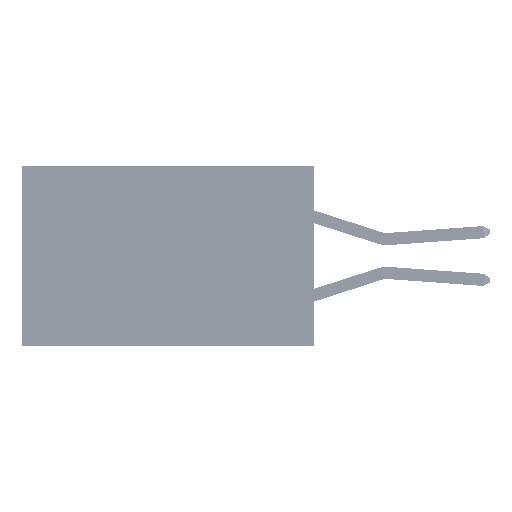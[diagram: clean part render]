
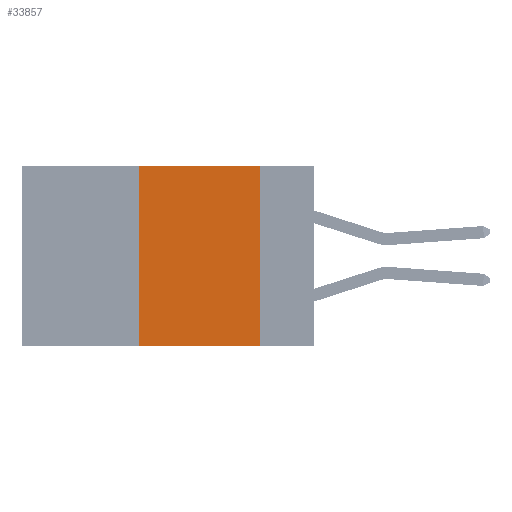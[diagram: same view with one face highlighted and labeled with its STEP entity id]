
A CAD part, left-side view. The second image highlights one B-rep face of the part: STEP entity #33857.
In plain terms, the highlighted planar face has unit normal (-1, 0, 0).
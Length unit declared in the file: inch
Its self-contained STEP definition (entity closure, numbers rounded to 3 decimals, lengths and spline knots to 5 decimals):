
#4185 = LINE ( 'NONE', #24525, #13109 ) ;
#5312 = VECTOR ( 'NONE', #49430, 39.37008 ) ;
#6240 = CARTESIAN_POINT ( 'NONE',  ( 0., 0.11, 0. ) ) ;
#9006 = ORIENTED_EDGE ( 'NONE', *, *, #12312, .T. ) ;
#10486 = EDGE_CURVE ( 'NONE', #29280, #26717, #4185, .T. ) ;
#10810 = EDGE_CURVE ( 'NONE', #26717, #48323, #37036, .T. ) ;
#11540 = DIRECTION ( 'NONE',  ( 1., 0., 0. ) ) ;
#12204 = VECTOR ( 'NONE', #24354, 39.37008 ) ;
#12312 = EDGE_CURVE ( 'NONE', #29280, #48264, #26581, .T. ) ;
#13109 = VECTOR ( 'NONE', #35706, 39.37008 ) ;
#14360 = CARTESIAN_POINT ( 'NONE',  ( 0., 0.11, 0. ) ) ;
#15136 = FACE_OUTER_BOUND ( 'NONE', #15821, .T. ) ;
#15810 = EDGE_CURVE ( 'NONE', #48323, #48264, #21415, .T. ) ;
#15821 = EDGE_LOOP ( 'NONE', ( #18045, #40813, #42378, #9006 ) ) ;
#18045 = ORIENTED_EDGE ( 'NONE', *, *, #15810, .F. ) ;
#20361 = CARTESIAN_POINT ( 'NONE',  ( 0., 0.36, 0. ) ) ;
#21415 = LINE ( 'NONE', #6240, #42325 ) ;
#23355 = CARTESIAN_POINT ( 'NONE',  ( 0., 0.6, -0.37 ) ) ;
#24354 = DIRECTION ( 'NONE',  ( 0., -1., 0. ) ) ;
#24525 = CARTESIAN_POINT ( 'NONE',  ( 0., 0.36, 0. ) ) ;
#24885 = CARTESIAN_POINT ( 'NONE',  ( 0., 0.11, -0.37 ) ) ;
#26581 = LINE ( 'NONE', #23355, #12204 ) ;
#26717 = VERTEX_POINT ( 'NONE', #20361 ) ;
#29280 = VERTEX_POINT ( 'NONE', #29823 ) ;
#29823 = CARTESIAN_POINT ( 'NONE',  ( 0., 0.36, -0.37 ) ) ;
#30083 = AXIS2_PLACEMENT_3D ( 'NONE', #37840, #11540, #30618 ) ;
#30618 = DIRECTION ( 'NONE',  ( 0., 0., -1. ) ) ;
#32639 = DIRECTION ( 'NONE',  ( 0., 0., -1. ) ) ;
#33857 = ADVANCED_FACE ( 'NONE', ( #15136 ), #40845, .F. ) ;
#35706 = DIRECTION ( 'NONE',  ( 0., 0., 1. ) ) ;
#37036 = LINE ( 'NONE', #45572, #5312 ) ;
#37840 = CARTESIAN_POINT ( 'NONE',  ( 0., 0.6, 0. ) ) ;
#40813 = ORIENTED_EDGE ( 'NONE', *, *, #10810, .F. ) ;
#40845 = PLANE ( 'NONE',  #30083 ) ;
#42325 = VECTOR ( 'NONE', #32639, 39.37008 ) ;
#42378 = ORIENTED_EDGE ( 'NONE', *, *, #10486, .F. ) ;
#45572 = CARTESIAN_POINT ( 'NONE',  ( 0., 0.6, 0. ) ) ;
#48264 = VERTEX_POINT ( 'NONE', #24885 ) ;
#48323 = VERTEX_POINT ( 'NONE', #14360 ) ;
#49430 = DIRECTION ( 'NONE',  ( 0., -1., 0. ) ) ;
